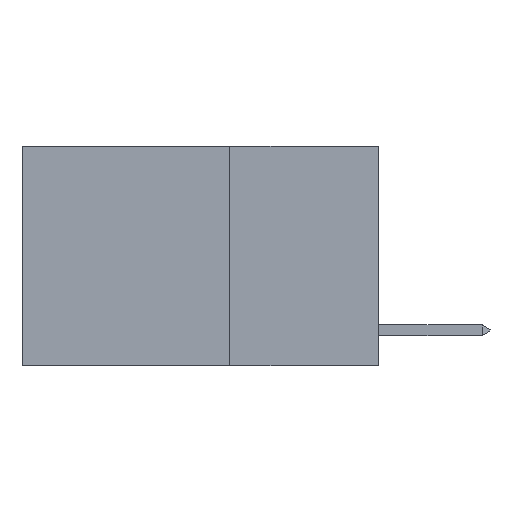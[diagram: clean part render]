
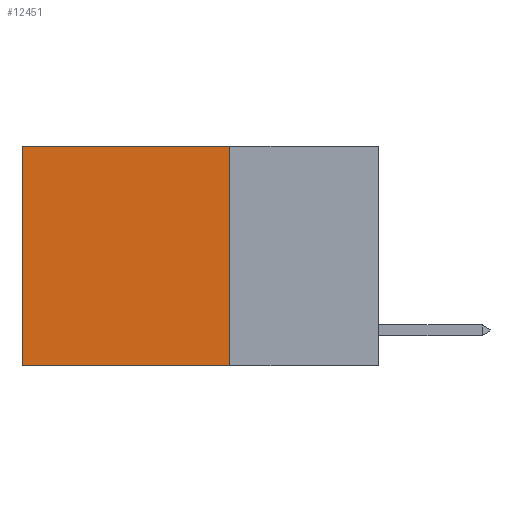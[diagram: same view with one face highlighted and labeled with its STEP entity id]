
A CAD part, left-side view. The second image highlights one B-rep face of the part: STEP entity #12451.
In plain terms, the highlighted planar face has unit normal (-1, 0, 0).
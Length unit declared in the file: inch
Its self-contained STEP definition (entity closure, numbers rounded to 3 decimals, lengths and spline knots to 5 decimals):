
#210 = VECTOR ( 'NONE', #18232, 39.37008 ) ;
#462 = LINE ( 'NONE', #22798, #11303 ) ;
#2415 = CARTESIAN_POINT ( 'NONE',  ( 0.2625, 0.6, 0. ) ) ;
#2959 = FACE_OUTER_BOUND ( 'NONE', #23952, .T. ) ;
#5101 = CARTESIAN_POINT ( 'NONE',  ( 0.2625, 0.25, 0. ) ) ;
#6159 = CARTESIAN_POINT ( 'NONE',  ( 0.2625, 0.25, 0. ) ) ;
#6907 = VERTEX_POINT ( 'NONE', #5101 ) ;
#7376 = VERTEX_POINT ( 'NONE', #2415 ) ;
#7734 = ORIENTED_EDGE ( 'NONE', *, *, #18144, .T. ) ;
#8068 = LINE ( 'NONE', #20030, #18120 ) ;
#9347 = CARTESIAN_POINT ( 'NONE',  ( 0.2625, 0.25, 0. ) ) ;
#10603 = EDGE_CURVE ( 'NONE', #12152, #17063, #462, .T. ) ;
#10771 = DIRECTION ( 'NONE',  ( 0., 1., 0. ) ) ;
#11032 = DIRECTION ( 'NONE',  ( 0., 0., -1. ) ) ;
#11303 = VECTOR ( 'NONE', #10771, 39.37008 ) ;
#11697 = LINE ( 'NONE', #6159, #210 ) ;
#12152 = VERTEX_POINT ( 'NONE', #12437 ) ;
#12437 = CARTESIAN_POINT ( 'NONE',  ( 0.2625, 0.25, -0.37 ) ) ;
#12451 = ADVANCED_FACE ( 'NONE', ( #2959 ), #23386, .F. ) ;
#12695 = EDGE_CURVE ( 'NONE', #6907, #12152, #8068, .T. ) ;
#13388 = DIRECTION ( 'NONE',  ( 0., 0., -1. ) ) ;
#14522 = ORIENTED_EDGE ( 'NONE', *, *, #12695, .F. ) ;
#15143 = ORIENTED_EDGE ( 'NONE', *, *, #10603, .F. ) ;
#17063 = VERTEX_POINT ( 'NONE', #22928 ) ;
#17089 = AXIS2_PLACEMENT_3D ( 'NONE', #9347, #25421, #13388 ) ;
#18120 = VECTOR ( 'NONE', #22058, 39.37008 ) ;
#18144 = EDGE_CURVE ( 'NONE', #6907, #7376, #11697, .T. ) ;
#18232 = DIRECTION ( 'NONE',  ( 0., 1., 0. ) ) ;
#20030 = CARTESIAN_POINT ( 'NONE',  ( 0.2625, 0.25, 0. ) ) ;
#20748 = ORIENTED_EDGE ( 'NONE', *, *, #21925, .T. ) ;
#21925 = EDGE_CURVE ( 'NONE', #7376, #17063, #24632, .T. ) ;
#22058 = DIRECTION ( 'NONE',  ( 0., 0., -1. ) ) ;
#22798 = CARTESIAN_POINT ( 'NONE',  ( 0.2625, 0.25, -0.37 ) ) ;
#22928 = CARTESIAN_POINT ( 'NONE',  ( 0.2625, 0.6, -0.37 ) ) ;
#23386 = PLANE ( 'NONE',  #17089 ) ;
#23952 = EDGE_LOOP ( 'NONE', ( #20748, #15143, #14522, #7734 ) ) ;
#23999 = VECTOR ( 'NONE', #11032, 39.37008 ) ;
#24632 = LINE ( 'NONE', #25169, #23999 ) ;
#25169 = CARTESIAN_POINT ( 'NONE',  ( 0.2625, 0.6, 0. ) ) ;
#25421 = DIRECTION ( 'NONE',  ( 1., 0., 0. ) ) ;
